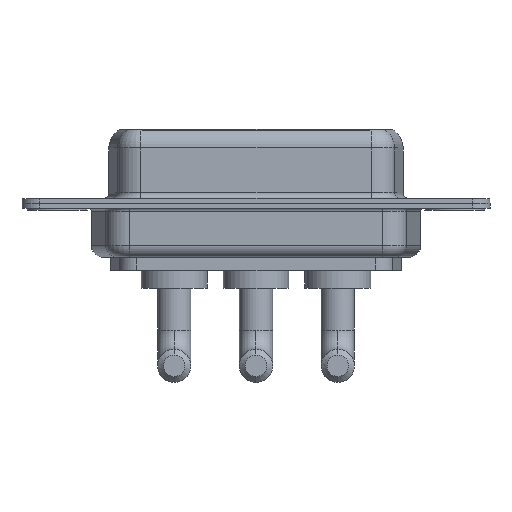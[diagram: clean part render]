
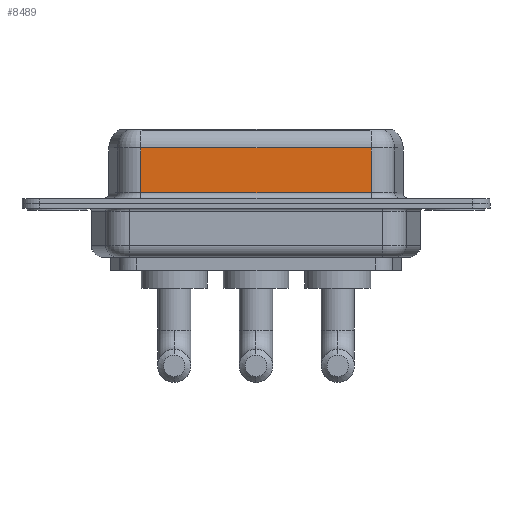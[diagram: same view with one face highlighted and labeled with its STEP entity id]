
A CAD part, front view. The second image highlights one B-rep face of the part: STEP entity #8489.
In plain terms, the highlighted planar face has unit normal (0, -1, 0).
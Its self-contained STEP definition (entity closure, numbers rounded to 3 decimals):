
#108 = EDGE_CURVE ( 'NONE', #6595, #1853, #7445, .T. ) ;
#251 = DIRECTION ( 'NONE',  ( 0., 1., 0. ) ) ;
#691 = CARTESIAN_POINT ( 'NONE',  ( 26.287, -3.95, 6.4 ) ) ;
#741 = CARTESIAN_POINT ( 'NONE',  ( 7.013, -3.95, 6.4 ) ) ;
#907 = EDGE_CURVE ( 'NONE', #1853, #6415, #10562, .T. ) ;
#1047 = FACE_OUTER_BOUND ( 'NONE', #3740, .T. ) ;
#1448 = VERTEX_POINT ( 'NONE', #6760 ) ;
#1853 = VERTEX_POINT ( 'NONE', #8245 ) ;
#2131 = LINE ( 'NONE', #9478, #5545 ) ;
#2185 = DIRECTION ( 'NONE',  ( -1., 0., 0. ) ) ;
#2588 = VECTOR ( 'NONE', #9066, 1000. ) ;
#3238 = DIRECTION ( 'NONE',  ( 0., 0., -1. ) ) ;
#3316 = CARTESIAN_POINT ( 'NONE',  ( 7.013, -3.95, 4.65 ) ) ;
#3510 = DIRECTION ( 'NONE',  ( 0., 0., 1. ) ) ;
#3740 = EDGE_LOOP ( 'NONE', ( #10208, #9188, #5507, #8613 ) ) ;
#4255 = VECTOR ( 'NONE', #3238, 1000. ) ;
#5428 = LINE ( 'NONE', #691, #9796 ) ;
#5507 = ORIENTED_EDGE ( 'NONE', *, *, #108, .T. ) ;
#5533 = AXIS2_PLACEMENT_3D ( 'NONE', #9210, #251, #3510 ) ;
#5545 = VECTOR ( 'NONE', #2185, 1000. ) ;
#6415 = VERTEX_POINT ( 'NONE', #8765 ) ;
#6595 = VERTEX_POINT ( 'NONE', #3316 ) ;
#6760 = CARTESIAN_POINT ( 'NONE',  ( 26.287, -3.95, 4.65 ) ) ;
#7239 = EDGE_CURVE ( 'NONE', #1448, #6595, #2131, .T. ) ;
#7411 = CARTESIAN_POINT ( 'NONE',  ( 26.287, -3.95, 0.9 ) ) ;
#7445 = LINE ( 'NONE', #741, #4255 ) ;
#7557 = PLANE ( 'NONE',  #5533 ) ;
#8187 = EDGE_CURVE ( 'NONE', #1448, #6415, #5428, .T. ) ;
#8245 = CARTESIAN_POINT ( 'NONE',  ( 7.013, -3.95, 0.9 ) ) ;
#8489 = ADVANCED_FACE ( 'NONE', ( #1047 ), #7557, .F. ) ;
#8613 = ORIENTED_EDGE ( 'NONE', *, *, #907, .T. ) ;
#8699 = DIRECTION ( 'NONE',  ( 0., 0., -1. ) ) ;
#8765 = CARTESIAN_POINT ( 'NONE',  ( 26.287, -3.95, 0.9 ) ) ;
#9066 = DIRECTION ( 'NONE',  ( 1., 0., 0. ) ) ;
#9188 = ORIENTED_EDGE ( 'NONE', *, *, #7239, .T. ) ;
#9210 = CARTESIAN_POINT ( 'NONE',  ( 26.287, -3.95, 6.4 ) ) ;
#9478 = CARTESIAN_POINT ( 'NONE',  ( 26.287, -3.95, 4.65 ) ) ;
#9796 = VECTOR ( 'NONE', #8699, 1000. ) ;
#10208 = ORIENTED_EDGE ( 'NONE', *, *, #8187, .F. ) ;
#10562 = LINE ( 'NONE', #7411, #2588 ) ;
